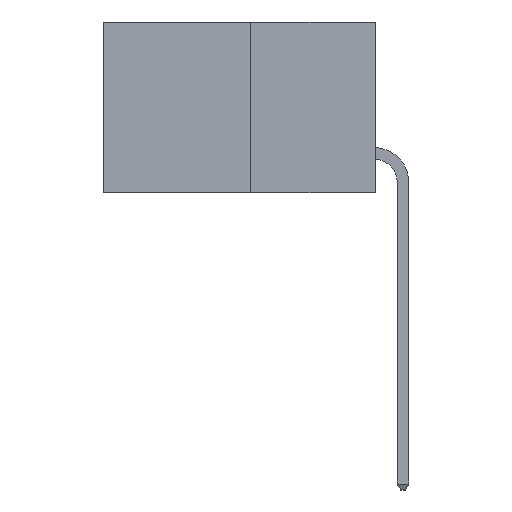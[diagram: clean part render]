
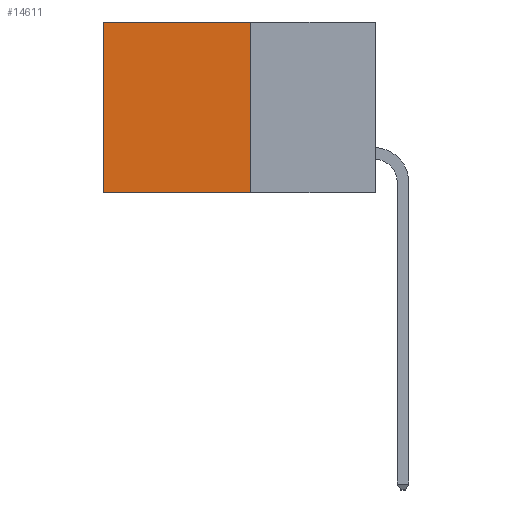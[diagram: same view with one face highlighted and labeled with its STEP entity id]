
A CAD part, left-side view. The second image highlights one B-rep face of the part: STEP entity #14611.
In plain terms, the highlighted planar face has unit normal (-1, 0, 0).
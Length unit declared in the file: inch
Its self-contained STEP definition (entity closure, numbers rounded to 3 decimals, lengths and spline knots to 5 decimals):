
#202 = LINE ( 'NONE', #13080, #7617 ) ;
#1765 = ORIENTED_EDGE ( 'NONE', *, *, #11721, .T. ) ;
#1939 = PLANE ( 'NONE',  #7365 ) ;
#2112 = CARTESIAN_POINT ( 'NONE',  ( 0.277, 0.59, -0.37 ) ) ;
#3479 = VECTOR ( 'NONE', #3573, 39.37008 ) ;
#3573 = DIRECTION ( 'NONE',  ( 0., 1., 0. ) ) ;
#3596 = DIRECTION ( 'NONE',  ( 0., 0., -1. ) ) ;
#4135 = FACE_OUTER_BOUND ( 'NONE', #18785, .T. ) ;
#4525 = CARTESIAN_POINT ( 'NONE',  ( 0.277, 0.27, 0. ) ) ;
#4976 = ORIENTED_EDGE ( 'NONE', *, *, #13979, .F. ) ;
#5437 = LINE ( 'NONE', #2112, #12402 ) ;
#6357 = VERTEX_POINT ( 'NONE', #10026 ) ;
#6410 = EDGE_CURVE ( 'NONE', #10475, #16189, #202, .T. ) ;
#7055 = ORIENTED_EDGE ( 'NONE', *, *, #6410, .F. ) ;
#7365 = AXIS2_PLACEMENT_3D ( 'NONE', #12287, #16684, #7879 ) ;
#7491 = DIRECTION ( 'NONE',  ( 0., 1., 0. ) ) ;
#7613 = CARTESIAN_POINT ( 'NONE',  ( 0.277, 0.27, -0.37 ) ) ;
#7617 = VECTOR ( 'NONE', #10158, 39.37008 ) ;
#7879 = DIRECTION ( 'NONE',  ( 0., 0., -1. ) ) ;
#8328 = LINE ( 'NONE', #12438, #3479 ) ;
#8419 = VERTEX_POINT ( 'NONE', #10086 ) ;
#10026 = CARTESIAN_POINT ( 'NONE',  ( 0.277, 0.59, 0. ) ) ;
#10086 = CARTESIAN_POINT ( 'NONE',  ( 0.277, 0.59, -0.37 ) ) ;
#10100 = ORIENTED_EDGE ( 'NONE', *, *, #14484, .T. ) ;
#10158 = DIRECTION ( 'NONE',  ( 0., 0., -1. ) ) ;
#10372 = VECTOR ( 'NONE', #7491, 39.37008 ) ;
#10475 = VERTEX_POINT ( 'NONE', #14155 ) ;
#10868 = LINE ( 'NONE', #4525, #10372 ) ;
#11721 = EDGE_CURVE ( 'NONE', #6357, #8419, #5437, .T. ) ;
#12287 = CARTESIAN_POINT ( 'NONE',  ( 0.277, 0.27, -0.37 ) ) ;
#12402 = VECTOR ( 'NONE', #3596, 39.37008 ) ;
#12438 = CARTESIAN_POINT ( 'NONE',  ( 0.277, 0.27, -0.37 ) ) ;
#13080 = CARTESIAN_POINT ( 'NONE',  ( 0.277, 0.27, -0.37 ) ) ;
#13979 = EDGE_CURVE ( 'NONE', #16189, #8419, #8328, .T. ) ;
#14155 = CARTESIAN_POINT ( 'NONE',  ( 0.277, 0.27, 0. ) ) ;
#14484 = EDGE_CURVE ( 'NONE', #10475, #6357, #10868, .T. ) ;
#14611 = ADVANCED_FACE ( 'NONE', ( #4135 ), #1939, .F. ) ;
#16189 = VERTEX_POINT ( 'NONE', #7613 ) ;
#16684 = DIRECTION ( 'NONE',  ( 1., 0., 0. ) ) ;
#18785 = EDGE_LOOP ( 'NONE', ( #1765, #4976, #7055, #10100 ) ) ;
